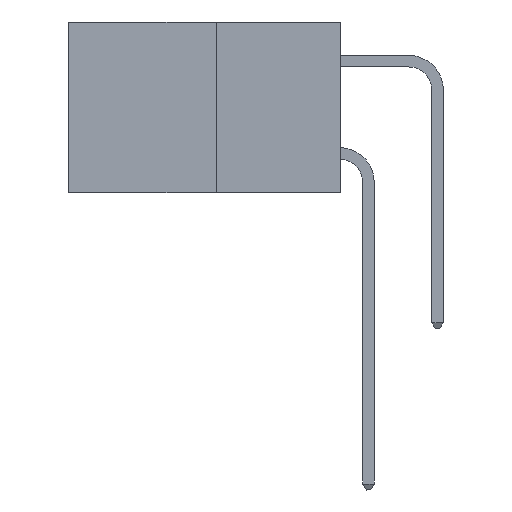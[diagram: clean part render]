
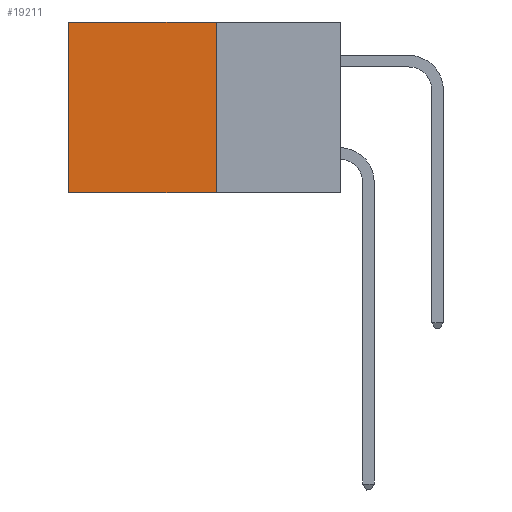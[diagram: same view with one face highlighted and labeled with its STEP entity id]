
A CAD part, left-side view. The second image highlights one B-rep face of the part: STEP entity #19211.
In plain terms, the highlighted planar face has unit normal (-1, 0, 0).
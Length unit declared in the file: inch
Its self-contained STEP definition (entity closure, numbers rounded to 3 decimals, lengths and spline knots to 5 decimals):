
#1461 = DIRECTION ( 'NONE',  ( 0., 0., -1. ) ) ;
#1710 = ORIENTED_EDGE ( 'NONE', *, *, #25381, .T. ) ;
#1852 = ORIENTED_EDGE ( 'NONE', *, *, #21821, .F. ) ;
#1856 = EDGE_CURVE ( 'NONE', #10797, #8618, #25413, .T. ) ;
#1929 = PLANE ( 'NONE',  #9555 ) ;
#4476 = FACE_OUTER_BOUND ( 'NONE', #25039, .T. ) ;
#5028 = LINE ( 'NONE', #16808, #9693 ) ;
#5552 = CARTESIAN_POINT ( 'NONE',  ( 0.277, 0.59, -0.37 ) ) ;
#5937 = DIRECTION ( 'NONE',  ( 1., 0., 0. ) ) ;
#6183 = CARTESIAN_POINT ( 'NONE',  ( 0.277, 0.27, 0. ) ) ;
#7770 = ORIENTED_EDGE ( 'NONE', *, *, #19734, .T. ) ;
#8618 = VERTEX_POINT ( 'NONE', #5552 ) ;
#9317 = DIRECTION ( 'NONE',  ( 0., 0., -1. ) ) ;
#9555 = AXIS2_PLACEMENT_3D ( 'NONE', #17878, #5937, #19870 ) ;
#9693 = VECTOR ( 'NONE', #18808, 39.37008 ) ;
#9722 = VERTEX_POINT ( 'NONE', #13203 ) ;
#10371 = CARTESIAN_POINT ( 'NONE',  ( 0.277, 0.27, -0.37 ) ) ;
#10797 = VERTEX_POINT ( 'NONE', #10371 ) ;
#11317 = CARTESIAN_POINT ( 'NONE',  ( 0.277, 0.59, -0.37 ) ) ;
#12380 = CARTESIAN_POINT ( 'NONE',  ( 0.277, 0.27, -0.37 ) ) ;
#12480 = VECTOR ( 'NONE', #1461, 39.37008 ) ;
#13203 = CARTESIAN_POINT ( 'NONE',  ( 0.277, 0.59, 0. ) ) ;
#13395 = CARTESIAN_POINT ( 'NONE',  ( 0.277, 0.27, -0.37 ) ) ;
#13734 = DIRECTION ( 'NONE',  ( 0., 1., 0. ) ) ;
#14381 = ORIENTED_EDGE ( 'NONE', *, *, #1856, .F. ) ;
#14798 = VECTOR ( 'NONE', #13734, 39.37008 ) ;
#16808 = CARTESIAN_POINT ( 'NONE',  ( 0.277, 0.27, 0. ) ) ;
#17766 = LINE ( 'NONE', #13395, #12480 ) ;
#17878 = CARTESIAN_POINT ( 'NONE',  ( 0.277, 0.27, -0.37 ) ) ;
#18808 = DIRECTION ( 'NONE',  ( 0., 1., 0. ) ) ;
#19211 = ADVANCED_FACE ( 'NONE', ( #4476 ), #1929, .F. ) ;
#19734 = EDGE_CURVE ( 'NONE', #9722, #8618, #23751, .T. ) ;
#19870 = DIRECTION ( 'NONE',  ( 0., 0., -1. ) ) ;
#21821 = EDGE_CURVE ( 'NONE', #25753, #10797, #17766, .T. ) ;
#23131 = VECTOR ( 'NONE', #9317, 39.37008 ) ;
#23751 = LINE ( 'NONE', #11317, #23131 ) ;
#25039 = EDGE_LOOP ( 'NONE', ( #7770, #14381, #1852, #1710 ) ) ;
#25381 = EDGE_CURVE ( 'NONE', #25753, #9722, #5028, .T. ) ;
#25413 = LINE ( 'NONE', #12380, #14798 ) ;
#25753 = VERTEX_POINT ( 'NONE', #6183 ) ;
